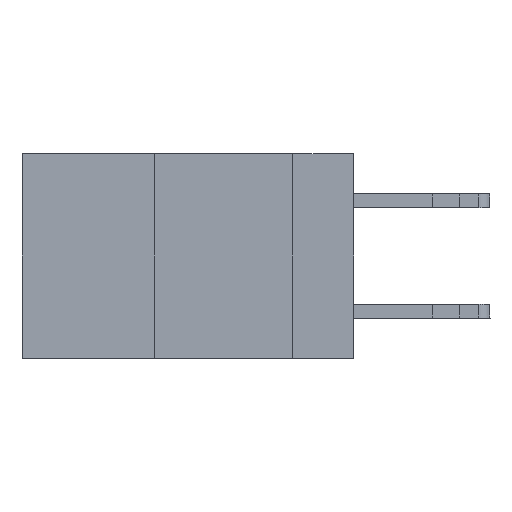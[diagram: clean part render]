
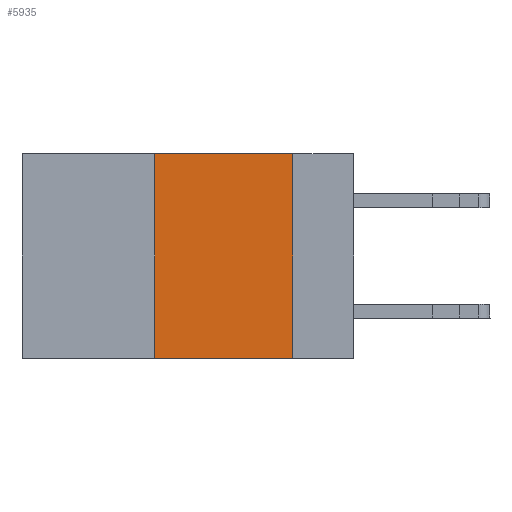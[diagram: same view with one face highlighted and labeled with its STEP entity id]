
A CAD part, left-side view. The second image highlights one B-rep face of the part: STEP entity #5935.
In plain terms, the highlighted planar face has unit normal (-1, 0, 0).
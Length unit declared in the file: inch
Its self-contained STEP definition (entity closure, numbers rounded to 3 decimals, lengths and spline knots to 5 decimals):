
#524 = CARTESIAN_POINT ( 'NONE',  ( 0., 0.6, 0. ) ) ;
#1481 = FACE_OUTER_BOUND ( 'NONE', #13516, .T. ) ;
#1660 = EDGE_CURVE ( 'NONE', #13438, #5565, #11304, .T. ) ;
#3382 = ORIENTED_EDGE ( 'NONE', *, *, #1660, .T. ) ;
#3524 = DIRECTION ( 'NONE',  ( 0., 0., -1. ) ) ;
#3587 = CARTESIAN_POINT ( 'NONE',  ( 0., 0.11, 0. ) ) ;
#3665 = DIRECTION ( 'NONE',  ( 0., 0., -1. ) ) ;
#3722 = EDGE_CURVE ( 'NONE', #13084, #5565, #11909, .T. ) ;
#3857 = LINE ( 'NONE', #16106, #19156 ) ;
#5565 = VERTEX_POINT ( 'NONE', #16216 ) ;
#5935 = ADVANCED_FACE ( 'NONE', ( #1481 ), #16949, .F. ) ;
#8186 = CARTESIAN_POINT ( 'NONE',  ( 0., 0.6, 0. ) ) ;
#8282 = ORIENTED_EDGE ( 'NONE', *, *, #3722, .F. ) ;
#8386 = EDGE_CURVE ( 'NONE', #9976, #13084, #14068, .T. ) ;
#9207 = CARTESIAN_POINT ( 'NONE',  ( 0., 0.11, 0. ) ) ;
#9976 = VERTEX_POINT ( 'NONE', #10693 ) ;
#10530 = ORIENTED_EDGE ( 'NONE', *, *, #16110, .F. ) ;
#10640 = VECTOR ( 'NONE', #18512, 39.37008 ) ;
#10693 = CARTESIAN_POINT ( 'NONE',  ( 0., 0.36, 0. ) ) ;
#10781 = ORIENTED_EDGE ( 'NONE', *, *, #8386, .F. ) ;
#10992 = VECTOR ( 'NONE', #3524, 39.37008 ) ;
#11304 = LINE ( 'NONE', #11735, #18638 ) ;
#11566 = CARTESIAN_POINT ( 'NONE',  ( 0., 0.36, -0.37 ) ) ;
#11735 = CARTESIAN_POINT ( 'NONE',  ( 0., 0.6, -0.37 ) ) ;
#11909 = LINE ( 'NONE', #3587, #10992 ) ;
#12658 = DIRECTION ( 'NONE',  ( 1., 0., 0. ) ) ;
#13084 = VERTEX_POINT ( 'NONE', #9207 ) ;
#13438 = VERTEX_POINT ( 'NONE', #11566 ) ;
#13516 = EDGE_LOOP ( 'NONE', ( #8282, #10781, #10530, #3382 ) ) ;
#14068 = LINE ( 'NONE', #8186, #10640 ) ;
#14291 = AXIS2_PLACEMENT_3D ( 'NONE', #524, #12658, #3665 ) ;
#15673 = DIRECTION ( 'NONE',  ( 0., -1., 0. ) ) ;
#16106 = CARTESIAN_POINT ( 'NONE',  ( 0., 0.36, 0. ) ) ;
#16110 = EDGE_CURVE ( 'NONE', #13438, #9976, #3857, .T. ) ;
#16216 = CARTESIAN_POINT ( 'NONE',  ( 0., 0.11, -0.37 ) ) ;
#16949 = PLANE ( 'NONE',  #14291 ) ;
#17560 = DIRECTION ( 'NONE',  ( 0., 0., 1. ) ) ;
#18512 = DIRECTION ( 'NONE',  ( 0., -1., 0. ) ) ;
#18638 = VECTOR ( 'NONE', #15673, 39.37008 ) ;
#19156 = VECTOR ( 'NONE', #17560, 39.37008 ) ;
